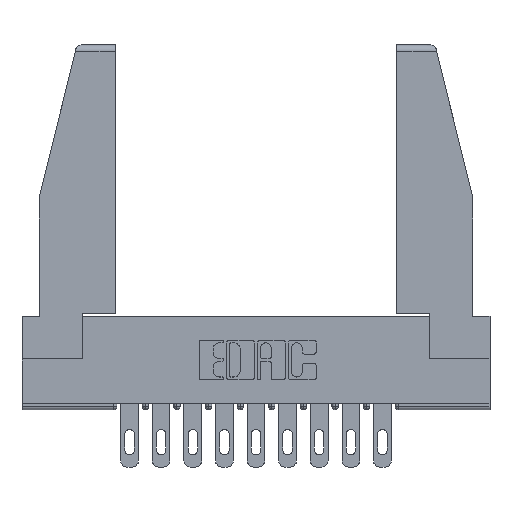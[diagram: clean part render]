
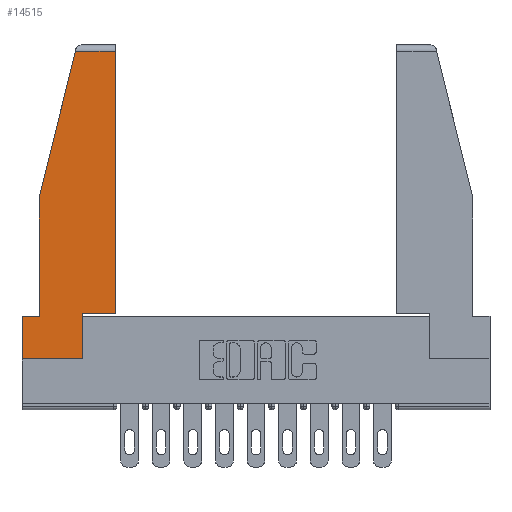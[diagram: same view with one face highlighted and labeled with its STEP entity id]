
A CAD part, top view. The second image highlights one B-rep face of the part: STEP entity #14515.
In plain terms, the highlighted planar face has unit normal (0, 0, 1).
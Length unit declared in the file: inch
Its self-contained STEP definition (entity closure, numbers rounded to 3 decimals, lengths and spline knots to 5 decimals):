
#316 = VERTEX_POINT ( 'NONE', #11027 ) ;
#367 = ORIENTED_EDGE ( 'NONE', *, *, #1267, .T. ) ;
#483 = CARTESIAN_POINT ( 'NONE',  ( 0.086, 0.8, 0. ) ) ;
#893 = ORIENTED_EDGE ( 'NONE', *, *, #10189, .T. ) ;
#922 = VERTEX_POINT ( 'NONE', #9832 ) ;
#1095 = DIRECTION ( 'NONE',  ( 1., 0., 0. ) ) ;
#1175 = VECTOR ( 'NONE', #12237, 39.37008 ) ;
#1267 = EDGE_CURVE ( 'NONE', #7095, #316, #14295, .T. ) ;
#1358 = CARTESIAN_POINT ( 'NONE',  ( 0.297, 0., 0. ) ) ;
#1649 = CARTESIAN_POINT ( 'NONE',  ( 0., 0., 0. ) ) ;
#1651 = CARTESIAN_POINT ( 'NONE',  ( 0., 0.21, 0. ) ) ;
#1854 = LINE ( 'NONE', #6546, #6198 ) ;
#2036 = VECTOR ( 'NONE', #10952, 39.37008 ) ;
#2111 = CARTESIAN_POINT ( 'NONE',  ( 0., 0.21, 0. ) ) ;
#2281 = EDGE_CURVE ( 'NONE', #6968, #5765, #3948, .T. ) ;
#2312 = CARTESIAN_POINT ( 'NONE',  ( 0.461, 0.223, 0. ) ) ;
#2529 = CARTESIAN_POINT ( 'NONE',  ( 0., 0., 0. ) ) ;
#2871 = CARTESIAN_POINT ( 'NONE',  ( 0., 0.21, 0. ) ) ;
#2907 = DIRECTION ( 'NONE',  ( 0., 1., 0. ) ) ;
#2921 = EDGE_LOOP ( 'NONE', ( #5804, #9168, #7342, #367, #14441, #4053, #14446, #11046, #893 ) ) ;
#3095 = EDGE_CURVE ( 'NONE', #5765, #11143, #4891, .T. ) ;
#3184 = VECTOR ( 'NONE', #14699, 39.37008 ) ;
#3948 = LINE ( 'NONE', #2871, #1175 ) ;
#4053 = ORIENTED_EDGE ( 'NONE', *, *, #2281, .T. ) ;
#4398 = LINE ( 'NONE', #2111, #12068 ) ;
#4891 = LINE ( 'NONE', #2529, #5063 ) ;
#5063 = VECTOR ( 'NONE', #13362, 39.37008 ) ;
#5327 = EDGE_CURVE ( 'NONE', #922, #7095, #7367, .T. ) ;
#5755 = PLANE ( 'NONE',  #13046 ) ;
#5765 = VERTEX_POINT ( 'NONE', #1649 ) ;
#5804 = ORIENTED_EDGE ( 'NONE', *, *, #9273, .T. ) ;
#6198 = VECTOR ( 'NONE', #2907, 39.37008 ) ;
#6327 = CARTESIAN_POINT ( 'NONE',  ( 0.297, 0., 0. ) ) ;
#6546 = CARTESIAN_POINT ( 'NONE',  ( 0.461, 0.223, 0. ) ) ;
#6952 = EDGE_CURVE ( 'NONE', #7257, #922, #8431, .T. ) ;
#6968 = VERTEX_POINT ( 'NONE', #1651 ) ;
#7095 = VERTEX_POINT ( 'NONE', #483 ) ;
#7257 = VERTEX_POINT ( 'NONE', #13156 ) ;
#7342 = ORIENTED_EDGE ( 'NONE', *, *, #5327, .T. ) ;
#7367 = LINE ( 'NONE', #8455, #2036 ) ;
#7518 = EDGE_CURVE ( 'NONE', #11143, #11083, #8728, .T. ) ;
#8070 = DIRECTION ( 'NONE',  ( 1., 0., 0. ) ) ;
#8431 = LINE ( 'NONE', #13172, #15046 ) ;
#8438 = VECTOR ( 'NONE', #1095, 39.37008 ) ;
#8455 = CARTESIAN_POINT ( 'NONE',  ( 0.271, 1.55, 0. ) ) ;
#8728 = LINE ( 'NONE', #6327, #3184 ) ;
#9168 = ORIENTED_EDGE ( 'NONE', *, *, #6952, .T. ) ;
#9273 = EDGE_CURVE ( 'NONE', #10516, #7257, #1854, .T. ) ;
#9393 = FACE_OUTER_BOUND ( 'NONE', #2921, .T. ) ;
#9551 = DIRECTION ( 'NONE',  ( 0., 0., 1. ) ) ;
#9812 = CARTESIAN_POINT ( 'NONE',  ( 0.086, 0.8, 0. ) ) ;
#9832 = CARTESIAN_POINT ( 'NONE',  ( 0.2636, 1.52, 0. ) ) ;
#10189 = EDGE_CURVE ( 'NONE', #11083, #10516, #10524, .T. ) ;
#10516 = VERTEX_POINT ( 'NONE', #2312 ) ;
#10524 = LINE ( 'NONE', #15177, #8438 ) ;
#10724 = CARTESIAN_POINT ( 'NONE',  ( 0., 0., 0. ) ) ;
#10952 = DIRECTION ( 'NONE',  ( -0.239, -0.971, 0. ) ) ;
#11027 = CARTESIAN_POINT ( 'NONE',  ( 0.086, 0.21, 0. ) ) ;
#11046 = ORIENTED_EDGE ( 'NONE', *, *, #7518, .T. ) ;
#11083 = VERTEX_POINT ( 'NONE', #13894 ) ;
#11143 = VERTEX_POINT ( 'NONE', #1358 ) ;
#11386 = DIRECTION ( 'NONE',  ( -1., 0., 0. ) ) ;
#11993 = DIRECTION ( 'NONE',  ( -1., 0., 0. ) ) ;
#12068 = VECTOR ( 'NONE', #11386, 39.37008 ) ;
#12123 = DIRECTION ( 'NONE',  ( 0., -1., 0. ) ) ;
#12237 = DIRECTION ( 'NONE',  ( 0., -1., 0. ) ) ;
#13046 = AXIS2_PLACEMENT_3D ( 'NONE', #10724, #9551, #8070 ) ;
#13156 = CARTESIAN_POINT ( 'NONE',  ( 0.461, 1.52, 0. ) ) ;
#13172 = CARTESIAN_POINT ( 'NONE',  ( 0., 1.52, 0. ) ) ;
#13362 = DIRECTION ( 'NONE',  ( 1., 0., 0. ) ) ;
#13513 = EDGE_CURVE ( 'NONE', #316, #6968, #4398, .T. ) ;
#13894 = CARTESIAN_POINT ( 'NONE',  ( 0.297, 0.223, 0. ) ) ;
#14295 = LINE ( 'NONE', #9812, #14625 ) ;
#14441 = ORIENTED_EDGE ( 'NONE', *, *, #13513, .T. ) ;
#14446 = ORIENTED_EDGE ( 'NONE', *, *, #3095, .T. ) ;
#14515 = ADVANCED_FACE ( 'NONE', ( #9393 ), #5755, .T. ) ;
#14625 = VECTOR ( 'NONE', #12123, 39.37008 ) ;
#14699 = DIRECTION ( 'NONE',  ( 0., 1., 0. ) ) ;
#15046 = VECTOR ( 'NONE', #11993, 39.37008 ) ;
#15177 = CARTESIAN_POINT ( 'NONE',  ( 0.297, 0.223, 0. ) ) ;
